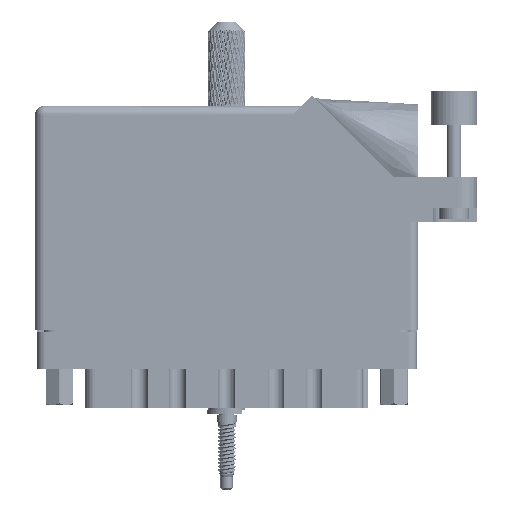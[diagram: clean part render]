
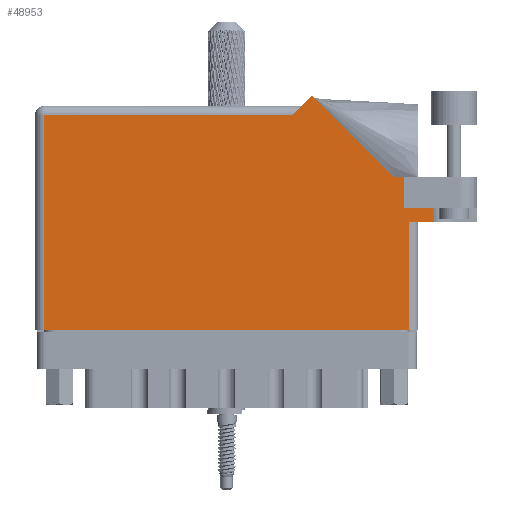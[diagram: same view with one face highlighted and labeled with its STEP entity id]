
A CAD part, front view. The second image highlights one B-rep face of the part: STEP entity #48953.
In plain terms, the highlighted face is planar.
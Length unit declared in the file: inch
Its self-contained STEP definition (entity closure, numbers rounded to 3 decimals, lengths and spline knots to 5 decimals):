
#1246 = CARTESIAN_POINT ( 'NONE',  ( 0., 1.53, 0. ) ) ;
#2563 = EDGE_CURVE ( 'NONE', #13725, #42491, #105192, .T. ) ;
#3667 = EDGE_CURVE ( 'NONE', #28343, #13725, #118877, .T. ) ;
#5763 = VECTOR ( 'NONE', #31189, 39.37008 ) ;
#10785 = VECTOR ( 'NONE', #111746, 39.37008 ) ;
#11190 = CARTESIAN_POINT ( 'NONE',  ( 1.819, 1.53, 0. ) ) ;
#11237 = PLANE ( 'NONE',  #14458 ) ;
#11390 = ORIENTED_EDGE ( 'NONE', *, *, #2563, .T. ) ;
#11614 = LINE ( 'NONE', #106128, #24052 ) ;
#12102 = DIRECTION ( 'NONE',  ( -1., 0., 0. ) ) ;
#12761 = ORIENTED_EDGE ( 'NONE', *, *, #3667, .T. ) ;
#13725 = VERTEX_POINT ( 'NONE', #44569 ) ;
#13919 = LINE ( 'NONE', #82751, #10785 ) ;
#14458 = AXIS2_PLACEMENT_3D ( 'NONE', #1246, #110401, #12102 ) ;
#15510 = DIRECTION ( 'NONE',  ( -0.707, 0.707, 0. ) ) ;
#16340 = LINE ( 'NONE', #112922, #50292 ) ;
#18497 = CARTESIAN_POINT ( 'NONE',  ( 0.062, 0., 0. ) ) ;
#18988 = LINE ( 'NONE', #65499, #65439 ) ;
#19992 = EDGE_CURVE ( 'NONE', #91462, #28343, #16340, .T. ) ;
#21950 = CARTESIAN_POINT ( 'NONE',  ( 2.512, 0.831, 0. ) ) ;
#24052 = VECTOR ( 'NONE', #117741, 39.37008 ) ;
#24786 = VERTEX_POINT ( 'NONE', #75520 ) ;
#26966 = VERTEX_POINT ( 'NONE', #38693 ) ;
#28343 = VERTEX_POINT ( 'NONE', #85075 ) ;
#29000 = EDGE_CURVE ( 'NONE', #73691, #87835, #31813, .T. ) ;
#30250 = DIRECTION ( 'NONE',  ( 0., -1., 0. ) ) ;
#31044 = DIRECTION ( 'NONE',  ( 1., 0., 0. ) ) ;
#31189 = DIRECTION ( 'NONE',  ( -0.707, -0.707, 0. ) ) ;
#31813 = LINE ( 'NONE', #77385, #48772 ) ;
#36344 = VERTEX_POINT ( 'NONE', #42037 ) ;
#38451 = DIRECTION ( 'NONE',  ( 0., -1., 0. ) ) ;
#38693 = CARTESIAN_POINT ( 'NONE',  ( 2.55, 0.737, 0. ) ) ;
#38894 = VECTOR ( 'NONE', #73423, 39.37008 ) ;
#39585 = CARTESIAN_POINT ( 'NONE',  ( 0., 1.468, 0. ) ) ;
#40445 = DIRECTION ( 'NONE',  ( -1., 0., 0. ) ) ;
#42037 = CARTESIAN_POINT ( 'NONE',  ( 2.55, 0., 0. ) ) ;
#42491 = VERTEX_POINT ( 'NONE', #124585 ) ;
#43284 = ORIENTED_EDGE ( 'NONE', *, *, #19992, .T. ) ;
#44569 = CARTESIAN_POINT ( 'NONE',  ( 1.757, 1.468, 0. ) ) ;
#48307 = EDGE_CURVE ( 'NONE', #73691, #90069, #49054, .T. ) ;
#48772 = VECTOR ( 'NONE', #85686, 39.37008 ) ;
#48953 = ADVANCED_FACE ( 'NONE', ( #103236 ), #11237, .F. ) ;
#49054 = LINE ( 'NONE', #109362, #79996 ) ;
#50292 = VECTOR ( 'NONE', #15510, 39.37008 ) ;
#51166 = LINE ( 'NONE', #88767, #100877 ) ;
#53188 = EDGE_CURVE ( 'NONE', #26966, #81964, #18988, .T. ) ;
#55978 = DIRECTION ( 'NONE',  ( 1., 0., 0. ) ) ;
#58756 = EDGE_LOOP ( 'NONE', ( #123081, #106435, #105939, #86471, #126777, #91647, #92902, #43284, #12761, #11390, #58894 ) ) ;
#58894 = ORIENTED_EDGE ( 'NONE', *, *, #104412, .T. ) ;
#60073 = EDGE_CURVE ( 'NONE', #36344, #26966, #11614, .T. ) ;
#64720 = CARTESIAN_POINT ( 'NONE',  ( 0., 0., 0. ) ) ;
#65439 = VECTOR ( 'NONE', #55978, 39.37008 ) ;
#65499 = CARTESIAN_POINT ( 'NONE',  ( 2.612, 0.737, 0. ) ) ;
#70131 = LINE ( 'NONE', #18497, #73282 ) ;
#71035 = EDGE_CURVE ( 'NONE', #90069, #81964, #51166, .T. ) ;
#73282 = VECTOR ( 'NONE', #38451, 39.37008 ) ;
#73423 = DIRECTION ( 'NONE',  ( 1., 0., 0. ) ) ;
#73691 = VERTEX_POINT ( 'NONE', #21950 ) ;
#75520 = CARTESIAN_POINT ( 'NONE',  ( 0.062, 0., 0. ) ) ;
#77385 = CARTESIAN_POINT ( 'NONE',  ( 2.512, 0.831, 0. ) ) ;
#79996 = VECTOR ( 'NONE', #31044, 39.37008 ) ;
#81355 = CARTESIAN_POINT ( 'NONE',  ( 2.7135, 0.831, 0. ) ) ;
#81964 = VERTEX_POINT ( 'NONE', #112459 ) ;
#82751 = CARTESIAN_POINT ( 'NONE',  ( 3.012, 1.044, 0. ) ) ;
#84678 = EDGE_CURVE ( 'NONE', #87835, #91462, #13919, .T. ) ;
#85075 = CARTESIAN_POINT ( 'NONE',  ( 1.88971, 1.60071, 0. ) ) ;
#85686 = DIRECTION ( 'NONE',  ( 0., 1., 0. ) ) ;
#86471 = ORIENTED_EDGE ( 'NONE', *, *, #71035, .F. ) ;
#87835 = VERTEX_POINT ( 'NONE', #91718 ) ;
#88767 = CARTESIAN_POINT ( 'NONE',  ( 2.7135, 1.16177, 0. ) ) ;
#90069 = VERTEX_POINT ( 'NONE', #81355 ) ;
#91462 = VERTEX_POINT ( 'NONE', #107782 ) ;
#91647 = ORIENTED_EDGE ( 'NONE', *, *, #29000, .T. ) ;
#91718 = CARTESIAN_POINT ( 'NONE',  ( 2.512, 1.044, 0. ) ) ;
#92902 = ORIENTED_EDGE ( 'NONE', *, *, #84678, .T. ) ;
#93103 = LINE ( 'NONE', #64720, #38894 ) ;
#100877 = VECTOR ( 'NONE', #30250, 39.37008 ) ;
#103236 = FACE_OUTER_BOUND ( 'NONE', #58756, .T. ) ;
#103677 = VECTOR ( 'NONE', #40445, 39.37008 ) ;
#104412 = EDGE_CURVE ( 'NONE', #42491, #24786, #70131, .T. ) ;
#105192 = LINE ( 'NONE', #39585, #103677 ) ;
#105939 = ORIENTED_EDGE ( 'NONE', *, *, #53188, .T. ) ;
#106128 = CARTESIAN_POINT ( 'NONE',  ( 2.55, 0.737, 0. ) ) ;
#106435 = ORIENTED_EDGE ( 'NONE', *, *, #60073, .T. ) ;
#106464 = EDGE_CURVE ( 'NONE', #24786, #36344, #93103, .T. ) ;
#107782 = CARTESIAN_POINT ( 'NONE',  ( 2.44642, 1.044, 0. ) ) ;
#109362 = CARTESIAN_POINT ( 'NONE',  ( 2.512, 0.831, 0. ) ) ;
#110401 = DIRECTION ( 'NONE',  ( 0., 0., -1. ) ) ;
#111746 = DIRECTION ( 'NONE',  ( -1., 0., 0. ) ) ;
#112459 = CARTESIAN_POINT ( 'NONE',  ( 2.7135, 0.737, 0. ) ) ;
#112922 = CARTESIAN_POINT ( 'NONE',  ( 2.44642, 1.044, 0. ) ) ;
#117741 = DIRECTION ( 'NONE',  ( 0., 1., 0. ) ) ;
#118877 = LINE ( 'NONE', #11190, #5763 ) ;
#123081 = ORIENTED_EDGE ( 'NONE', *, *, #106464, .T. ) ;
#124585 = CARTESIAN_POINT ( 'NONE',  ( 0.062, 1.468, 0. ) ) ;
#126777 = ORIENTED_EDGE ( 'NONE', *, *, #48307, .F. ) ;
